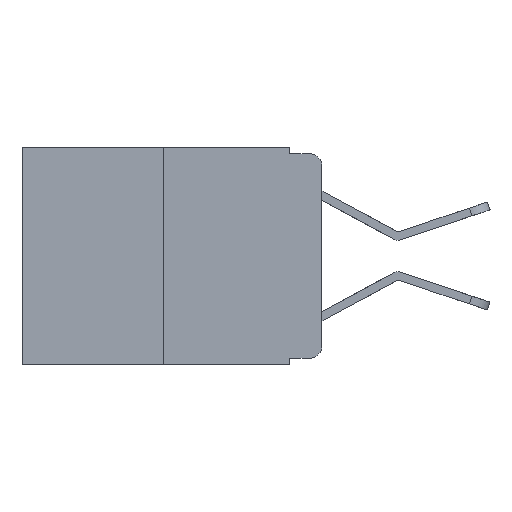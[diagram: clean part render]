
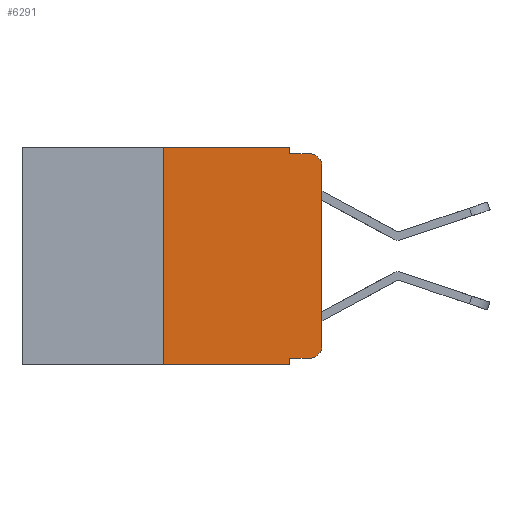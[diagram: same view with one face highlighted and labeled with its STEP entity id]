
A CAD part, left-side view. The second image highlights one B-rep face of the part: STEP entity #6291.
In plain terms, the highlighted planar face has unit normal (-1, 0, 0).
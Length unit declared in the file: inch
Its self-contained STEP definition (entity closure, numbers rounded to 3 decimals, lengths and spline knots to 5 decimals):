
#236 = DIRECTION ( 'NONE',  ( 0., -1., 0. ) ) ;
#617 = VERTEX_POINT ( 'NONE', #8986 ) ;
#855 = PLANE ( 'NONE',  #7522 ) ;
#942 = CARTESIAN_POINT ( 'NONE',  ( 0., 0., 0. ) ) ;
#961 = ORIENTED_EDGE ( 'NONE', *, *, #8451, .T. ) ;
#1030 = VECTOR ( 'NONE', #2078, 39.37008 ) ;
#1049 = CARTESIAN_POINT ( 'NONE',  ( 0., 0.25, 0. ) ) ;
#1129 = ORIENTED_EDGE ( 'NONE', *, *, #9975, .T. ) ;
#1294 = DIRECTION ( 'NONE',  ( 0., 0., 1. ) ) ;
#1414 = DIRECTION ( 'NONE',  ( 0., -1., 0. ) ) ;
#1458 = ORIENTED_EDGE ( 'NONE', *, *, #2873, .T. ) ;
#1598 = AXIS2_PLACEMENT_3D ( 'NONE', #6134, #6144, #4468 ) ;
#1607 = ORIENTED_EDGE ( 'NONE', *, *, #3409, .T. ) ;
#1688 = EDGE_CURVE ( 'NONE', #3192, #4850, #7893, .T. ) ;
#1772 = VERTEX_POINT ( 'NONE', #7289 ) ;
#1992 = ORIENTED_EDGE ( 'NONE', *, *, #4539, .F. ) ;
#1997 = ORIENTED_EDGE ( 'NONE', *, *, #9831, .F. ) ;
#2078 = DIRECTION ( 'NONE',  ( 0., -1., 0. ) ) ;
#2097 = VECTOR ( 'NONE', #2729, 39.37008 ) ;
#2103 = CARTESIAN_POINT ( 'NONE',  ( 0., 0.051, -0.01 ) ) ;
#2261 = ORIENTED_EDGE ( 'NONE', *, *, #3563, .T. ) ;
#2309 = VECTOR ( 'NONE', #2987, 39.37008 ) ;
#2396 = DIRECTION ( 'NONE',  ( 0., 0., -1. ) ) ;
#2400 = VECTOR ( 'NONE', #1414, 39.37008 ) ;
#2540 = ORIENTED_EDGE ( 'NONE', *, *, #1688, .F. ) ;
#2729 = DIRECTION ( 'NONE',  ( 0., 0., 1. ) ) ;
#2825 = ORIENTED_EDGE ( 'NONE', *, *, #9255, .F. ) ;
#2873 = EDGE_CURVE ( 'NONE', #7454, #1772, #5077, .T. ) ;
#2930 = CARTESIAN_POINT ( 'NONE',  ( 0., 0.051, 0. ) ) ;
#2987 = DIRECTION ( 'NONE',  ( 0., 0., -1. ) ) ;
#3136 = ORIENTED_EDGE ( 'NONE', *, *, #6202, .F. ) ;
#3183 = VERTEX_POINT ( 'NONE', #7331 ) ;
#3192 = VERTEX_POINT ( 'NONE', #7877 ) ;
#3324 = DIRECTION ( 'NONE',  ( 0., 0., -1. ) ) ;
#3405 = VERTEX_POINT ( 'NONE', #4514 ) ;
#3409 = EDGE_CURVE ( 'NONE', #3405, #7454, #6820, .T. ) ;
#3563 = EDGE_CURVE ( 'NONE', #9128, #617, #3848, .T. ) ;
#3670 = VECTOR ( 'NONE', #2396, 39.37008 ) ;
#3707 = LINE ( 'NONE', #5199, #5522 ) ;
#3848 = CIRCLE ( 'NONE', #4839, 0.02 ) ;
#3854 = VERTEX_POINT ( 'NONE', #6770 ) ;
#3900 = FACE_OUTER_BOUND ( 'NONE', #4804, .T. ) ;
#4468 = DIRECTION ( 'NONE',  ( 0., 0., -1. ) ) ;
#4473 = LINE ( 'NONE', #942, #2097 ) ;
#4514 = CARTESIAN_POINT ( 'NONE',  ( 0., 0.051, -0.333 ) ) ;
#4539 = EDGE_CURVE ( 'NONE', #3183, #3854, #8429, .T. ) ;
#4754 = CARTESIAN_POINT ( 'NONE',  ( 0., 0.051, 0. ) ) ;
#4804 = EDGE_LOOP ( 'NONE', ( #1129, #2261, #3136, #1992, #2825, #2540, #961, #1997, #1607, #1458 ) ) ;
#4821 = VECTOR ( 'NONE', #8784, 39.37008 ) ;
#4839 = AXIS2_PLACEMENT_3D ( 'NONE', #8184, #8030, #3324 ) ;
#4850 = VERTEX_POINT ( 'NONE', #1049 ) ;
#5077 = CIRCLE ( 'NONE', #1598, 0.02 ) ;
#5199 = CARTESIAN_POINT ( 'NONE',  ( 0., 0.473, -0.343 ) ) ;
#5522 = VECTOR ( 'NONE', #236, 39.37008 ) ;
#5670 = CARTESIAN_POINT ( 'NONE',  ( 0., 0.051, -0.343 ) ) ;
#6134 = CARTESIAN_POINT ( 'NONE',  ( 0., 0.02, -0.313 ) ) ;
#6144 = DIRECTION ( 'NONE',  ( -1., 0., 0. ) ) ;
#6202 = EDGE_CURVE ( 'NONE', #3854, #617, #7374, .T. ) ;
#6291 = ADVANCED_FACE ( 'NONE', ( #3900 ), #855, .F. ) ;
#6363 = VERTEX_POINT ( 'NONE', #5670 ) ;
#6770 = CARTESIAN_POINT ( 'NONE',  ( 0., 0.051, -0.01 ) ) ;
#6820 = LINE ( 'NONE', #9783, #4821 ) ;
#6949 = CARTESIAN_POINT ( 'NONE',  ( 0., 0.473, 0. ) ) ;
#7289 = CARTESIAN_POINT ( 'NONE',  ( 0., 0., -0.313 ) ) ;
#7302 = DIRECTION ( 'NONE',  ( 1., 0., 0. ) ) ;
#7331 = CARTESIAN_POINT ( 'NONE',  ( 0., 0.051, 0. ) ) ;
#7338 = DIRECTION ( 'NONE',  ( 0., 0., -1. ) ) ;
#7374 = LINE ( 'NONE', #2103, #1030 ) ;
#7454 = VERTEX_POINT ( 'NONE', #7739 ) ;
#7522 = AXIS2_PLACEMENT_3D ( 'NONE', #8430, #7302, #7338 ) ;
#7739 = CARTESIAN_POINT ( 'NONE',  ( 0., 0.02, -0.333 ) ) ;
#7877 = CARTESIAN_POINT ( 'NONE',  ( 0., 0.25, -0.343 ) ) ;
#7893 = LINE ( 'NONE', #9193, #8110 ) ;
#7943 = LINE ( 'NONE', #4754, #3670 ) ;
#8030 = DIRECTION ( 'NONE',  ( -1., 0., 0. ) ) ;
#8110 = VECTOR ( 'NONE', #1294, 39.37008 ) ;
#8184 = CARTESIAN_POINT ( 'NONE',  ( 0., 0.02, -0.03 ) ) ;
#8429 = LINE ( 'NONE', #2930, #2309 ) ;
#8430 = CARTESIAN_POINT ( 'NONE',  ( 0., 0.473, 0. ) ) ;
#8451 = EDGE_CURVE ( 'NONE', #3192, #6363, #3707, .T. ) ;
#8506 = LINE ( 'NONE', #6949, #2400 ) ;
#8784 = DIRECTION ( 'NONE',  ( 0., -1., 0. ) ) ;
#8965 = CARTESIAN_POINT ( 'NONE',  ( 0., 0., -0.03 ) ) ;
#8986 = CARTESIAN_POINT ( 'NONE',  ( 0., 0.02, -0.01 ) ) ;
#9128 = VERTEX_POINT ( 'NONE', #8965 ) ;
#9193 = CARTESIAN_POINT ( 'NONE',  ( 0., 0.25, 0. ) ) ;
#9255 = EDGE_CURVE ( 'NONE', #4850, #3183, #8506, .T. ) ;
#9783 = CARTESIAN_POINT ( 'NONE',  ( 0., 0.051, -0.333 ) ) ;
#9831 = EDGE_CURVE ( 'NONE', #3405, #6363, #7943, .T. ) ;
#9975 = EDGE_CURVE ( 'NONE', #1772, #9128, #4473, .T. ) ;
